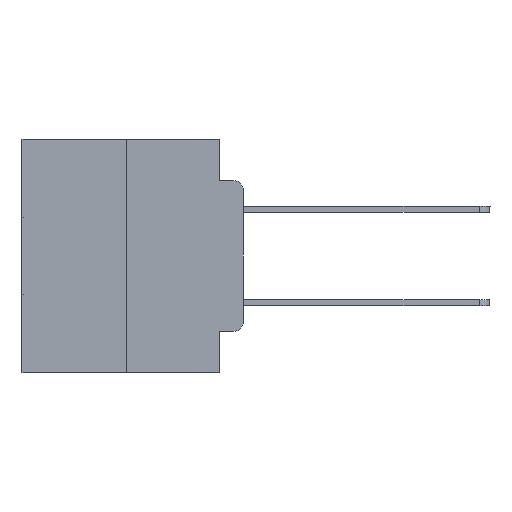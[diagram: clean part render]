
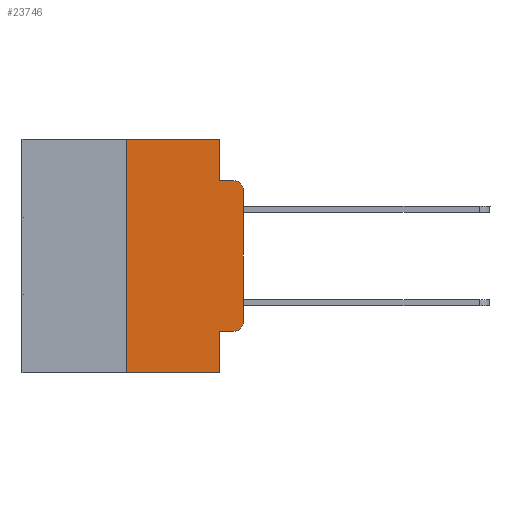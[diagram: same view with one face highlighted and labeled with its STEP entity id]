
A CAD part, left-side view. The second image highlights one B-rep face of the part: STEP entity #23746.
In plain terms, the highlighted planar face has unit normal (-1, 0, 0).
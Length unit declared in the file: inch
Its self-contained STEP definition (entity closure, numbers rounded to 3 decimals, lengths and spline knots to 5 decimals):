
#17 = EDGE_CURVE ( 'NONE', #25299, #16643, #18040, .T. ) ;
#520 = ORIENTED_EDGE ( 'NONE', *, *, #28479, .T. ) ;
#924 = ORIENTED_EDGE ( 'NONE', *, *, #17, .F. ) ;
#969 = ORIENTED_EDGE ( 'NONE', *, *, #3026, .F. ) ;
#1789 = VECTOR ( 'NONE', #6658, 39.37008 ) ;
#1966 = CARTESIAN_POINT ( 'NONE',  ( 0., 0.051, -0.4115 ) ) ;
#2061 = LINE ( 'NONE', #22485, #14261 ) ;
#2332 = VERTEX_POINT ( 'NONE', #13316 ) ;
#2351 = CARTESIAN_POINT ( 'NONE',  ( 0., 0.051, -0.4115 ) ) ;
#3026 = EDGE_CURVE ( 'NONE', #2332, #25299, #17333, .T. ) ;
#3088 = ORIENTED_EDGE ( 'NONE', *, *, #14065, .T. ) ;
#3314 = ORIENTED_EDGE ( 'NONE', *, *, #29877, .F. ) ;
#4618 = CARTESIAN_POINT ( 'NONE',  ( 0., 0., 0. ) ) ;
#4807 = DIRECTION ( 'NONE',  ( 0., 0., -1. ) ) ;
#5152 = LINE ( 'NONE', #11770, #16830 ) ;
#5430 = ORIENTED_EDGE ( 'NONE', *, *, #28388, .T. ) ;
#5561 = VERTEX_POINT ( 'NONE', #2351 ) ;
#5911 = ORIENTED_EDGE ( 'NONE', *, *, #6229, .F. ) ;
#6229 = EDGE_CURVE ( 'NONE', #16643, #29367, #21114, .T. ) ;
#6260 = CARTESIAN_POINT ( 'NONE',  ( 0., 0.473, 0. ) ) ;
#6627 = CARTESIAN_POINT ( 'NONE',  ( 0., 0.051, -0.0885 ) ) ;
#6658 = DIRECTION ( 'NONE',  ( 0., -1., 0. ) ) ;
#6877 = AXIS2_PLACEMENT_3D ( 'NONE', #12846, #8260, #24390 ) ;
#6940 = CARTESIAN_POINT ( 'NONE',  ( 0., 0.25, 0. ) ) ;
#7032 = DIRECTION ( 'NONE',  ( 0., 0., 1. ) ) ;
#7174 = DIRECTION ( 'NONE',  ( 0., -1., 0. ) ) ;
#7200 = CARTESIAN_POINT ( 'NONE',  ( 0., 0.051, 0. ) ) ;
#7492 = DIRECTION ( 'NONE',  ( 0., -1., 0. ) ) ;
#7802 = CARTESIAN_POINT ( 'NONE',  ( 0., 0.02, -0.3915 ) ) ;
#8112 = VERTEX_POINT ( 'NONE', #27900 ) ;
#8260 = DIRECTION ( 'NONE',  ( 1., 0., 0. ) ) ;
#9368 = EDGE_CURVE ( 'NONE', #29367, #21451, #16893, .T. ) ;
#9423 = CARTESIAN_POINT ( 'NONE',  ( 0., 0., -0.1085 ) ) ;
#9427 = AXIS2_PLACEMENT_3D ( 'NONE', #13061, #29022, #15393 ) ;
#10140 = DIRECTION ( 'NONE',  ( 0., 0., -1. ) ) ;
#10609 = DIRECTION ( 'NONE',  ( 0., 0., 1. ) ) ;
#10633 = CARTESIAN_POINT ( 'NONE',  ( 0., 0.051, 0. ) ) ;
#10734 = VECTOR ( 'NONE', #7492, 39.37008 ) ;
#11006 = DIRECTION ( 'NONE',  ( 0., 0., -1. ) ) ;
#11180 = VECTOR ( 'NONE', #10609, 39.37008 ) ;
#11327 = EDGE_LOOP ( 'NONE', ( #24613, #3088, #27692, #5911, #924, #969, #520, #3314, #5430, #13411 ) ) ;
#11770 = CARTESIAN_POINT ( 'NONE',  ( 0., 0.473, -0.5 ) ) ;
#12022 = AXIS2_PLACEMENT_3D ( 'NONE', #7802, #23926, #10140 ) ;
#12846 = CARTESIAN_POINT ( 'NONE',  ( 0., 0.473, 0. ) ) ;
#13061 = CARTESIAN_POINT ( 'NONE',  ( 0., 0.02, -0.1085 ) ) ;
#13316 = CARTESIAN_POINT ( 'NONE',  ( 0., 0.25, -0.5 ) ) ;
#13411 = ORIENTED_EDGE ( 'NONE', *, *, #26898, .T. ) ;
#14065 = EDGE_CURVE ( 'NONE', #28890, #21451, #22715, .T. ) ;
#14261 = VECTOR ( 'NONE', #11006, 39.37008 ) ;
#14412 = VECTOR ( 'NONE', #7032, 39.37008 ) ;
#15037 = EDGE_CURVE ( 'NONE', #21389, #28890, #21207, .T. ) ;
#15263 = CARTESIAN_POINT ( 'NONE',  ( 0., 0.25, 0. ) ) ;
#15393 = DIRECTION ( 'NONE',  ( 0., 0., -1. ) ) ;
#15841 = CARTESIAN_POINT ( 'NONE',  ( 0., 0.02, -0.0885 ) ) ;
#16643 = VERTEX_POINT ( 'NONE', #10633 ) ;
#16721 = CARTESIAN_POINT ( 'NONE',  ( 0., 0.051, -0.0885 ) ) ;
#16830 = VECTOR ( 'NONE', #7174, 39.37008 ) ;
#16893 = LINE ( 'NONE', #16721, #10734 ) ;
#17333 = LINE ( 'NONE', #15263, #11180 ) ;
#18040 = LINE ( 'NONE', #6260, #29410 ) ;
#20546 = FACE_OUTER_BOUND ( 'NONE', #11327, .T. ) ;
#21105 = LINE ( 'NONE', #1966, #1789 ) ;
#21114 = LINE ( 'NONE', #7200, #26499 ) ;
#21207 = LINE ( 'NONE', #4618, #14412 ) ;
#21389 = VERTEX_POINT ( 'NONE', #22365 ) ;
#21451 = VERTEX_POINT ( 'NONE', #15841 ) ;
#22096 = PLANE ( 'NONE',  #6877 ) ;
#22365 = CARTESIAN_POINT ( 'NONE',  ( 0., 0., -0.3915 ) ) ;
#22485 = CARTESIAN_POINT ( 'NONE',  ( 0., 0.051, 0. ) ) ;
#22715 = CIRCLE ( 'NONE', #9427, 0.02 ) ;
#23746 = ADVANCED_FACE ( 'NONE', ( #20546 ), #22096, .F. ) ;
#23926 = DIRECTION ( 'NONE',  ( -1., 0., 0. ) ) ;
#24390 = DIRECTION ( 'NONE',  ( 0., 0., -1. ) ) ;
#24613 = ORIENTED_EDGE ( 'NONE', *, *, #15037, .T. ) ;
#24685 = DIRECTION ( 'NONE',  ( 0., -1., 0. ) ) ;
#25299 = VERTEX_POINT ( 'NONE', #6940 ) ;
#26499 = VECTOR ( 'NONE', #4807, 39.37008 ) ;
#26898 = EDGE_CURVE ( 'NONE', #28406, #21389, #29957, .T. ) ;
#27493 = CARTESIAN_POINT ( 'NONE',  ( 0., 0.02, -0.4115 ) ) ;
#27692 = ORIENTED_EDGE ( 'NONE', *, *, #9368, .F. ) ;
#27900 = CARTESIAN_POINT ( 'NONE',  ( 0., 0.051, -0.5 ) ) ;
#28388 = EDGE_CURVE ( 'NONE', #5561, #28406, #21105, .T. ) ;
#28406 = VERTEX_POINT ( 'NONE', #27493 ) ;
#28479 = EDGE_CURVE ( 'NONE', #2332, #8112, #5152, .T. ) ;
#28890 = VERTEX_POINT ( 'NONE', #9423 ) ;
#29022 = DIRECTION ( 'NONE',  ( -1., 0., 0. ) ) ;
#29367 = VERTEX_POINT ( 'NONE', #6627 ) ;
#29410 = VECTOR ( 'NONE', #24685, 39.37008 ) ;
#29877 = EDGE_CURVE ( 'NONE', #5561, #8112, #2061, .T. ) ;
#29957 = CIRCLE ( 'NONE', #12022, 0.02 ) ;
